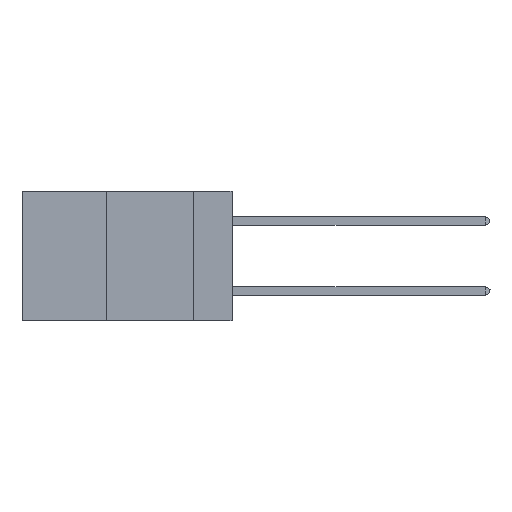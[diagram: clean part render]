
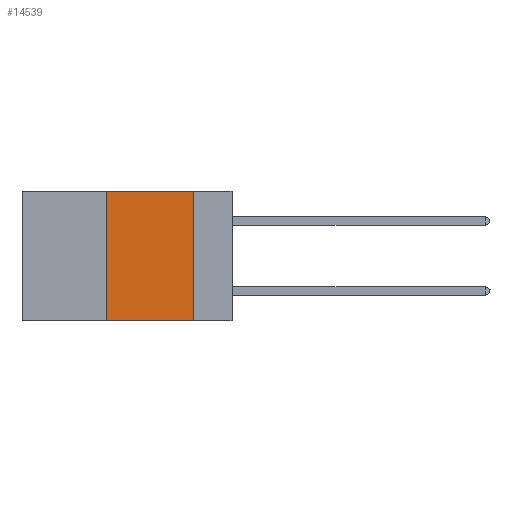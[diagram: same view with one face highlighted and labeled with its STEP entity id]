
A CAD part, left-side view. The second image highlights one B-rep face of the part: STEP entity #14539.
In plain terms, the highlighted planar face has unit normal (-1, 0, 0).
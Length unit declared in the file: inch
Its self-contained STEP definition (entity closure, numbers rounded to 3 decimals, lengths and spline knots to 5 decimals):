
#77 = LINE ( 'NONE', #6574, #9169 ) ;
#967 = ORIENTED_EDGE ( 'NONE', *, *, #13638, .F. ) ;
#1435 = FACE_OUTER_BOUND ( 'NONE', #5294, .T. ) ;
#1490 = VERTEX_POINT ( 'NONE', #13513 ) ;
#1851 = CARTESIAN_POINT ( 'NONE',  ( 0., 0.6, 0. ) ) ;
#2377 = CARTESIAN_POINT ( 'NONE',  ( 0., 0.6, -0.37 ) ) ;
#2844 = VERTEX_POINT ( 'NONE', #5837 ) ;
#5294 = EDGE_LOOP ( 'NONE', ( #967, #10899, #7880, #15011 ) ) ;
#5837 = CARTESIAN_POINT ( 'NONE',  ( 0., 0.36, 0. ) ) ;
#6574 = CARTESIAN_POINT ( 'NONE',  ( 0., 0.11, 0. ) ) ;
#6811 = DIRECTION ( 'NONE',  ( 0., -1., 0. ) ) ;
#7063 = DIRECTION ( 'NONE',  ( 0., 0., 1. ) ) ;
#7880 = ORIENTED_EDGE ( 'NONE', *, *, #12828, .F. ) ;
#8274 = PLANE ( 'NONE',  #14421 ) ;
#9169 = VECTOR ( 'NONE', #10570, 39.37008 ) ;
#9185 = VECTOR ( 'NONE', #9408, 39.37008 ) ;
#9408 = DIRECTION ( 'NONE',  ( 0., -1., 0. ) ) ;
#9414 = LINE ( 'NONE', #14798, #12673 ) ;
#9643 = DIRECTION ( 'NONE',  ( 1., 0., 0. ) ) ;
#10467 = VECTOR ( 'NONE', #6811, 39.37008 ) ;
#10528 = VERTEX_POINT ( 'NONE', #15089 ) ;
#10570 = DIRECTION ( 'NONE',  ( 0., 0., -1. ) ) ;
#10899 = ORIENTED_EDGE ( 'NONE', *, *, #11830, .F. ) ;
#11027 = CARTESIAN_POINT ( 'NONE',  ( 0., 0.36, -0.37 ) ) ;
#11196 = LINE ( 'NONE', #2377, #9185 ) ;
#11830 = EDGE_CURVE ( 'NONE', #2844, #10528, #13892, .T. ) ;
#12170 = DIRECTION ( 'NONE',  ( 0., 0., -1. ) ) ;
#12673 = VECTOR ( 'NONE', #7063, 39.37008 ) ;
#12828 = EDGE_CURVE ( 'NONE', #13462, #2844, #9414, .T. ) ;
#13243 = EDGE_CURVE ( 'NONE', #13462, #1490, #11196, .T. ) ;
#13462 = VERTEX_POINT ( 'NONE', #11027 ) ;
#13513 = CARTESIAN_POINT ( 'NONE',  ( 0., 0.11, -0.37 ) ) ;
#13638 = EDGE_CURVE ( 'NONE', #10528, #1490, #77, .T. ) ;
#13892 = LINE ( 'NONE', #1851, #10467 ) ;
#14421 = AXIS2_PLACEMENT_3D ( 'NONE', #15894, #9643, #12170 ) ;
#14539 = ADVANCED_FACE ( 'NONE', ( #1435 ), #8274, .F. ) ;
#14798 = CARTESIAN_POINT ( 'NONE',  ( 0., 0.36, 0. ) ) ;
#15011 = ORIENTED_EDGE ( 'NONE', *, *, #13243, .T. ) ;
#15089 = CARTESIAN_POINT ( 'NONE',  ( 0., 0.11, 0. ) ) ;
#15894 = CARTESIAN_POINT ( 'NONE',  ( 0., 0.6, 0. ) ) ;
